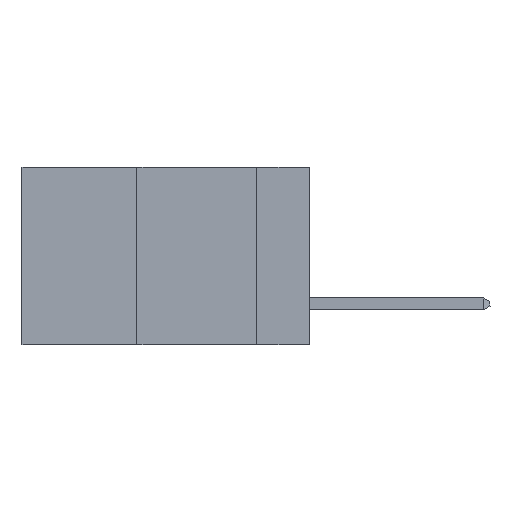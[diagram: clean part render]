
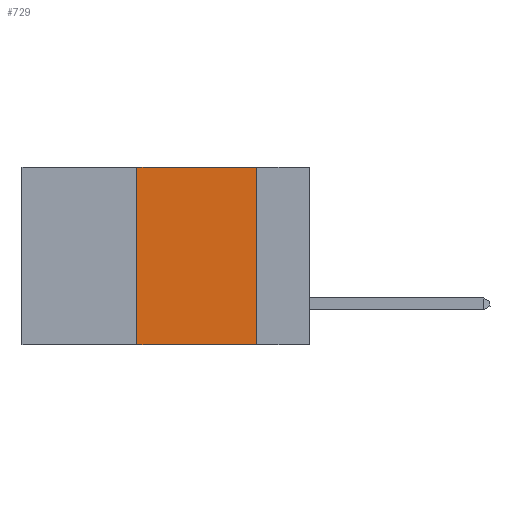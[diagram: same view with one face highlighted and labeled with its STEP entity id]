
A CAD part, left-side view. The second image highlights one B-rep face of the part: STEP entity #729.
In plain terms, the highlighted planar face has unit normal (-1, 0, 0).
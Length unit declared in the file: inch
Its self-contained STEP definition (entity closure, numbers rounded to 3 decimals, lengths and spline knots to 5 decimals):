
#45 = EDGE_CURVE ( 'NONE', #1379, #203, #2669, .T. ) ;
#203 = VERTEX_POINT ( 'NONE', #4053 ) ;
#582 = LINE ( 'NONE', #9839, #11116 ) ;
#617 = EDGE_CURVE ( 'NONE', #14150, #13969, #4015, .T. ) ;
#729 = ADVANCED_FACE ( 'NONE', ( #11509 ), #2133, .F. ) ;
#829 = LINE ( 'NONE', #11610, #4269 ) ;
#837 = CARTESIAN_POINT ( 'NONE',  ( 0., 0.6, 0. ) ) ;
#1379 = VERTEX_POINT ( 'NONE', #8734 ) ;
#1637 = ORIENTED_EDGE ( 'NONE', *, *, #8076, .F. ) ;
#2133 = PLANE ( 'NONE',  #6576 ) ;
#2188 = DIRECTION ( 'NONE',  ( 0., -1., 0. ) ) ;
#2669 = LINE ( 'NONE', #7601, #8669 ) ;
#4015 = LINE ( 'NONE', #15664, #6271 ) ;
#4053 = CARTESIAN_POINT ( 'NONE',  ( 0., 0.11, 0. ) ) ;
#4269 = VECTOR ( 'NONE', #12979, 39.37008 ) ;
#4424 = DIRECTION ( 'NONE',  ( 1., 0., 0. ) ) ;
#6271 = VECTOR ( 'NONE', #6877, 39.37008 ) ;
#6576 = AXIS2_PLACEMENT_3D ( 'NONE', #837, #4424, #9250 ) ;
#6579 = DIRECTION ( 'NONE',  ( 0., 0., 1. ) ) ;
#6877 = DIRECTION ( 'NONE',  ( 0., -1., 0. ) ) ;
#7601 = CARTESIAN_POINT ( 'NONE',  ( 0., 0.6, 0. ) ) ;
#8076 = EDGE_CURVE ( 'NONE', #203, #13969, #829, .T. ) ;
#8669 = VECTOR ( 'NONE', #2188, 39.37008 ) ;
#8721 = EDGE_CURVE ( 'NONE', #14150, #1379, #582, .T. ) ;
#8734 = CARTESIAN_POINT ( 'NONE',  ( 0., 0.36, 0. ) ) ;
#9250 = DIRECTION ( 'NONE',  ( 0., 0., -1. ) ) ;
#9455 = ORIENTED_EDGE ( 'NONE', *, *, #45, .F. ) ;
#9654 = CARTESIAN_POINT ( 'NONE',  ( 0., 0.11, -0.37 ) ) ;
#9839 = CARTESIAN_POINT ( 'NONE',  ( 0., 0.36, 0. ) ) ;
#10931 = ORIENTED_EDGE ( 'NONE', *, *, #8721, .F. ) ;
#11116 = VECTOR ( 'NONE', #6579, 39.37008 ) ;
#11509 = FACE_OUTER_BOUND ( 'NONE', #14064, .T. ) ;
#11610 = CARTESIAN_POINT ( 'NONE',  ( 0., 0.11, 0. ) ) ;
#12979 = DIRECTION ( 'NONE',  ( 0., 0., -1. ) ) ;
#13969 = VERTEX_POINT ( 'NONE', #9654 ) ;
#14064 = EDGE_LOOP ( 'NONE', ( #1637, #9455, #10931, #14633 ) ) ;
#14150 = VERTEX_POINT ( 'NONE', #15506 ) ;
#14633 = ORIENTED_EDGE ( 'NONE', *, *, #617, .T. ) ;
#15506 = CARTESIAN_POINT ( 'NONE',  ( 0., 0.36, -0.37 ) ) ;
#15664 = CARTESIAN_POINT ( 'NONE',  ( 0., 0.6, -0.37 ) ) ;
